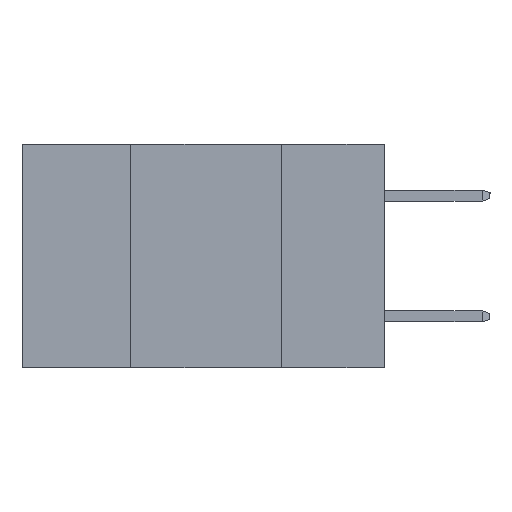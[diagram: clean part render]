
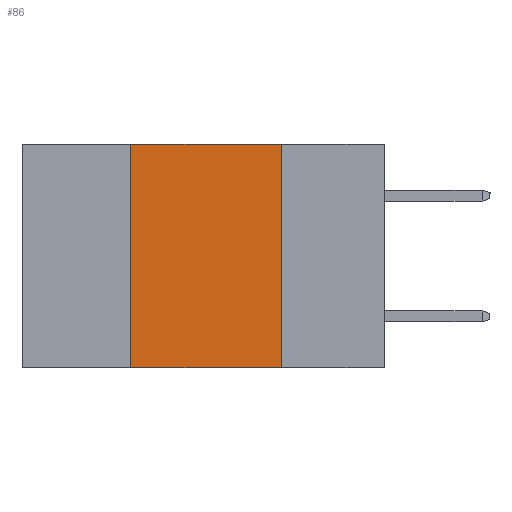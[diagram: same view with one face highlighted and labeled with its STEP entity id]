
A CAD part, left-side view. The second image highlights one B-rep face of the part: STEP entity #86.
In plain terms, the highlighted planar face has unit normal (-1, 0, 0).
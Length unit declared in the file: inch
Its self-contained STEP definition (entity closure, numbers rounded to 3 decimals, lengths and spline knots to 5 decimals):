
#86 = ADVANCED_FACE ( 'NONE', ( #1688 ), #4817, .F. ) ;
#220 = AXIS2_PLACEMENT_3D ( 'NONE', #3439, #4612, #8953 ) ;
#329 = EDGE_LOOP ( 'NONE', ( #10532, #12542, #7649, #10035 ) ) ;
#1688 = FACE_OUTER_BOUND ( 'NONE', #329, .T. ) ;
#3410 = VERTEX_POINT ( 'NONE', #5142 ) ;
#3439 = CARTESIAN_POINT ( 'NONE',  ( 0., 0.6, 0. ) ) ;
#3905 = CARTESIAN_POINT ( 'NONE',  ( 0., 0.6, -0.37 ) ) ;
#4612 = DIRECTION ( 'NONE',  ( 1., 0., 0. ) ) ;
#4817 = PLANE ( 'NONE',  #220 ) ;
#5142 = CARTESIAN_POINT ( 'NONE',  ( 0., 0.17, -0.37 ) ) ;
#5611 = LINE ( 'NONE', #10817, #11186 ) ;
#5734 = DIRECTION ( 'NONE',  ( 0., 0., 1. ) ) ;
#5781 = CARTESIAN_POINT ( 'NONE',  ( 0., 0.42, 0. ) ) ;
#6671 = VECTOR ( 'NONE', #5734, 39.37008 ) ;
#7140 = EDGE_CURVE ( 'NONE', #8606, #8847, #5611, .T. ) ;
#7649 = ORIENTED_EDGE ( 'NONE', *, *, #7811, .F. ) ;
#7811 = EDGE_CURVE ( 'NONE', #11800, #8606, #10874, .T. ) ;
#8293 = EDGE_CURVE ( 'NONE', #8847, #3410, #13330, .T. ) ;
#8606 = VERTEX_POINT ( 'NONE', #5781 ) ;
#8847 = VERTEX_POINT ( 'NONE', #9182 ) ;
#8866 = VECTOR ( 'NONE', #12235, 39.37008 ) ;
#8953 = DIRECTION ( 'NONE',  ( 0., 0., -1. ) ) ;
#8995 = CARTESIAN_POINT ( 'NONE',  ( 0., 0.42, -0.37 ) ) ;
#9182 = CARTESIAN_POINT ( 'NONE',  ( 0., 0.17, 0. ) ) ;
#9183 = DIRECTION ( 'NONE',  ( 0., -1., 0. ) ) ;
#10035 = ORIENTED_EDGE ( 'NONE', *, *, #11554, .T. ) ;
#10076 = LINE ( 'NONE', #3905, #11913 ) ;
#10532 = ORIENTED_EDGE ( 'NONE', *, *, #8293, .F. ) ;
#10817 = CARTESIAN_POINT ( 'NONE',  ( 0., 0.6, 0. ) ) ;
#10874 = LINE ( 'NONE', #8995, #6671 ) ;
#11186 = VECTOR ( 'NONE', #11819, 39.37008 ) ;
#11222 = CARTESIAN_POINT ( 'NONE',  ( 0., 0.17, -0.37 ) ) ;
#11554 = EDGE_CURVE ( 'NONE', #11800, #3410, #10076, .T. ) ;
#11800 = VERTEX_POINT ( 'NONE', #12554 ) ;
#11819 = DIRECTION ( 'NONE',  ( 0., -1., 0. ) ) ;
#11913 = VECTOR ( 'NONE', #9183, 39.37008 ) ;
#12235 = DIRECTION ( 'NONE',  ( 0., 0., -1. ) ) ;
#12542 = ORIENTED_EDGE ( 'NONE', *, *, #7140, .F. ) ;
#12554 = CARTESIAN_POINT ( 'NONE',  ( 0., 0.42, -0.37 ) ) ;
#13330 = LINE ( 'NONE', #11222, #8866 ) ;
